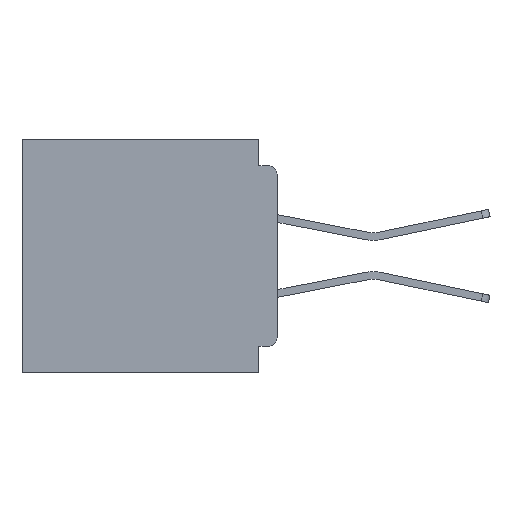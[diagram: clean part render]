
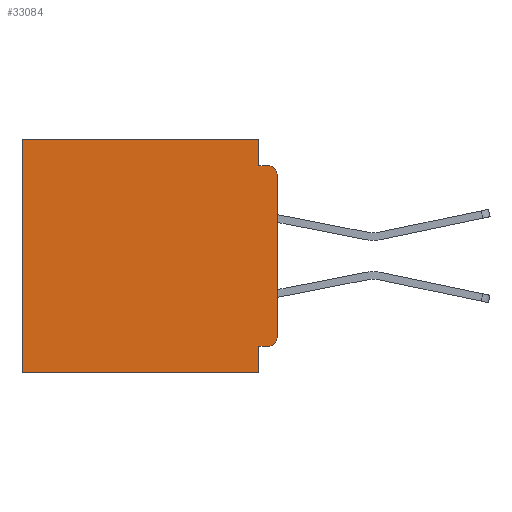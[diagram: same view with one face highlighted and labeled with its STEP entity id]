
A CAD part, left-side view. The second image highlights one B-rep face of the part: STEP entity #33084.
In plain terms, the highlighted planar face has unit normal (-1, 0, 0).
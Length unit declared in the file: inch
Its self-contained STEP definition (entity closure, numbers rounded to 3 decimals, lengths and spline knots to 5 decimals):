
#64 = CARTESIAN_POINT ( 'NONE',  ( 0.3, 0.031, -0.4 ) ) ;
#1370 = VECTOR ( 'NONE', #21460, 39.37008 ) ;
#1861 = VECTOR ( 'NONE', #11931, 39.37008 ) ;
#2813 = LINE ( 'NONE', #64, #1861 ) ;
#2966 = AXIS2_PLACEMENT_3D ( 'NONE', #9903, #30195, #12849 ) ;
#3288 = CARTESIAN_POINT ( 'NONE',  ( 0.3, 0.031, 0. ) ) ;
#3900 = PLANE ( 'NONE',  #2966 ) ;
#4328 = ORIENTED_EDGE ( 'NONE', *, *, #14779, .F. ) ;
#4346 = DIRECTION ( 'NONE',  ( 0., 0., -1. ) ) ;
#4554 = VERTEX_POINT ( 'NONE', #28593 ) ;
#4715 = VERTEX_POINT ( 'NONE', #30193 ) ;
#5822 = VECTOR ( 'NONE', #13192, 39.37008 ) ;
#6791 = CARTESIAN_POINT ( 'NONE',  ( 0.3, 0., -0.34 ) ) ;
#7459 = DIRECTION ( 'NONE',  ( -1., 0., 0. ) ) ;
#7932 = VERTEX_POINT ( 'NONE', #9737 ) ;
#8006 = CARTESIAN_POINT ( 'NONE',  ( 0.3, 0., -0.4 ) ) ;
#8384 = CARTESIAN_POINT ( 'NONE',  ( 0.3, 0.015, -0.355 ) ) ;
#8538 = DIRECTION ( 'NONE',  ( 0., 1., 0. ) ) ;
#8798 = VERTEX_POINT ( 'NONE', #25439 ) ;
#9591 = EDGE_CURVE ( 'NONE', #36145, #4554, #2813, .T. ) ;
#9737 = CARTESIAN_POINT ( 'NONE',  ( 0.3, 0.031, -0.045 ) ) ;
#9769 = DIRECTION ( 'NONE',  ( -1., 0., 0. ) ) ;
#9903 = CARTESIAN_POINT ( 'NONE',  ( 0.3, 0., -0.4 ) ) ;
#10259 = CARTESIAN_POINT ( 'NONE',  ( 0.3, 0.437, -0.4 ) ) ;
#10430 = ORIENTED_EDGE ( 'NONE', *, *, #9591, .F. ) ;
#11022 = DIRECTION ( 'NONE',  ( 0., 1., 0. ) ) ;
#11561 = EDGE_CURVE ( 'NONE', #17364, #7932, #23811, .T. ) ;
#11751 = VECTOR ( 'NONE', #11022, 39.37008 ) ;
#11931 = DIRECTION ( 'NONE',  ( 0., 0., -1. ) ) ;
#12185 = ORIENTED_EDGE ( 'NONE', *, *, #18774, .F. ) ;
#12355 = EDGE_CURVE ( 'NONE', #32141, #13892, #27337, .T. ) ;
#12773 = ORIENTED_EDGE ( 'NONE', *, *, #35599, .F. ) ;
#12849 = DIRECTION ( 'NONE',  ( 0., 0., -1. ) ) ;
#12955 = LINE ( 'NONE', #19062, #35103 ) ;
#12985 = CARTESIAN_POINT ( 'NONE',  ( 0.3, 0.031, 0. ) ) ;
#13192 = DIRECTION ( 'NONE',  ( 0., 0., -1. ) ) ;
#13892 = VERTEX_POINT ( 'NONE', #6791 ) ;
#14047 = ORIENTED_EDGE ( 'NONE', *, *, #24072, .T. ) ;
#14058 = VECTOR ( 'NONE', #8538, 39.37008 ) ;
#14189 = CARTESIAN_POINT ( 'NONE',  ( 0.3, 0.031, -0.355 ) ) ;
#14779 = EDGE_CURVE ( 'NONE', #4554, #8798, #33910, .T. ) ;
#15975 = CIRCLE ( 'NONE', #31363, 0.015 ) ;
#16518 = VERTEX_POINT ( 'NONE', #37479 ) ;
#17364 = VERTEX_POINT ( 'NONE', #12985 ) ;
#17511 = VERTEX_POINT ( 'NONE', #25172 ) ;
#17928 = VECTOR ( 'NONE', #20960, 39.37008 ) ;
#18537 = CARTESIAN_POINT ( 'NONE',  ( 0.3, 0., -0.045 ) ) ;
#18774 = EDGE_CURVE ( 'NONE', #4715, #13892, #12955, .T. ) ;
#19062 = CARTESIAN_POINT ( 'NONE',  ( 0.3, 0., -0.4 ) ) ;
#20960 = DIRECTION ( 'NONE',  ( 0., 0., -1. ) ) ;
#21460 = DIRECTION ( 'NONE',  ( 0., -1., 0. ) ) ;
#22333 = FACE_OUTER_BOUND ( 'NONE', #28326, .T. ) ;
#22366 = ORIENTED_EDGE ( 'NONE', *, *, #12355, .T. ) ;
#22584 = EDGE_CURVE ( 'NONE', #17364, #16518, #37063, .T. ) ;
#23049 = LINE ( 'NONE', #18537, #1370 ) ;
#23457 = CARTESIAN_POINT ( 'NONE',  ( 0.3, 0., 0. ) ) ;
#23485 = EDGE_CURVE ( 'NONE', #16518, #8798, #30028, .T. ) ;
#23811 = LINE ( 'NONE', #3288, #17928 ) ;
#24072 = EDGE_CURVE ( 'NONE', #4715, #17511, #15975, .T. ) ;
#24952 = ORIENTED_EDGE ( 'NONE', *, *, #23485, .T. ) ;
#24977 = CARTESIAN_POINT ( 'NONE',  ( 0.3, 0.015, -0.06 ) ) ;
#25172 = CARTESIAN_POINT ( 'NONE',  ( 0.3, 0.015, -0.045 ) ) ;
#25439 = CARTESIAN_POINT ( 'NONE',  ( 0.3, 0.437, -0.4 ) ) ;
#27171 = CARTESIAN_POINT ( 'NONE',  ( 0.3, 0.015, -0.34 ) ) ;
#27184 = EDGE_CURVE ( 'NONE', #7932, #17511, #23049, .T. ) ;
#27337 = CIRCLE ( 'NONE', #27348, 0.015 ) ;
#27348 = AXIS2_PLACEMENT_3D ( 'NONE', #27171, #9769, #30070 ) ;
#27884 = DIRECTION ( 'NONE',  ( 0., 0., -1. ) ) ;
#28109 = ORIENTED_EDGE ( 'NONE', *, *, #11561, .F. ) ;
#28326 = EDGE_LOOP ( 'NONE', ( #12185, #14047, #33020, #28109, #37471, #24952, #4328, #10430, #12773, #22366 ) ) ;
#28593 = CARTESIAN_POINT ( 'NONE',  ( 0.3, 0.031, -0.4 ) ) ;
#28655 = CARTESIAN_POINT ( 'NONE',  ( 0.3, 0., -0.355 ) ) ;
#29456 = VECTOR ( 'NONE', #32381, 39.37008 ) ;
#30028 = LINE ( 'NONE', #10259, #5822 ) ;
#30070 = DIRECTION ( 'NONE',  ( 0., 0., -1. ) ) ;
#30193 = CARTESIAN_POINT ( 'NONE',  ( 0.3, 0., -0.06 ) ) ;
#30195 = DIRECTION ( 'NONE',  ( 1., 0., 0. ) ) ;
#31363 = AXIS2_PLACEMENT_3D ( 'NONE', #24977, #7459, #27884 ) ;
#32141 = VERTEX_POINT ( 'NONE', #8384 ) ;
#32381 = DIRECTION ( 'NONE',  ( 0., 1., 0. ) ) ;
#33020 = ORIENTED_EDGE ( 'NONE', *, *, #27184, .F. ) ;
#33084 = ADVANCED_FACE ( 'NONE', ( #22333 ), #3900, .F. ) ;
#33910 = LINE ( 'NONE', #8006, #11751 ) ;
#35103 = VECTOR ( 'NONE', #4346, 39.37008 ) ;
#35599 = EDGE_CURVE ( 'NONE', #32141, #36145, #37035, .T. ) ;
#36145 = VERTEX_POINT ( 'NONE', #14189 ) ;
#37035 = LINE ( 'NONE', #28655, #14058 ) ;
#37063 = LINE ( 'NONE', #23457, #29456 ) ;
#37471 = ORIENTED_EDGE ( 'NONE', *, *, #22584, .T. ) ;
#37479 = CARTESIAN_POINT ( 'NONE',  ( 0.3, 0.437, 0. ) ) ;
